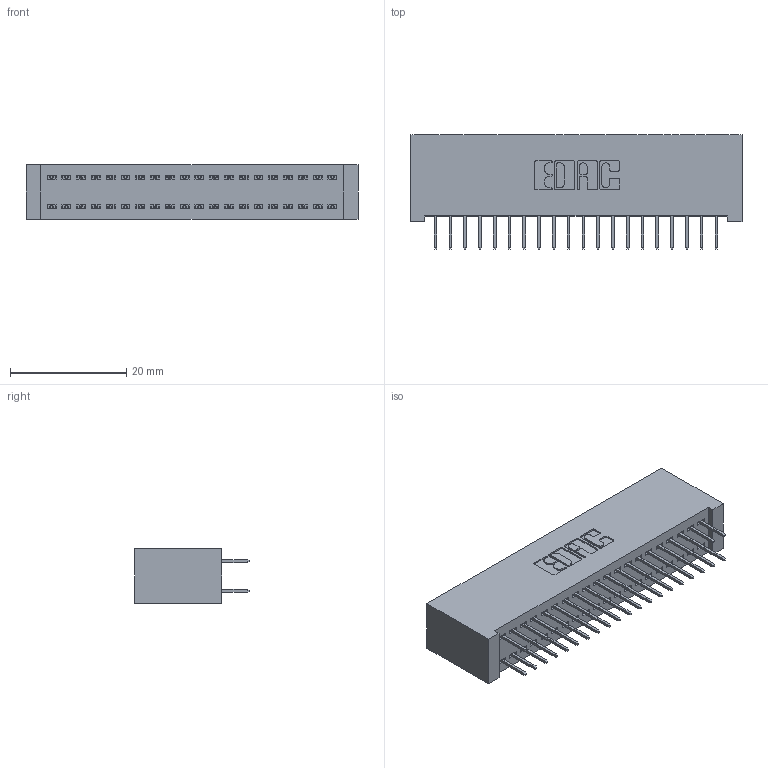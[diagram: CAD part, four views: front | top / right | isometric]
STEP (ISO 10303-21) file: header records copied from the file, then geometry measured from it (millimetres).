
FILE_DESCRIPTION (( 'STEP AP203' ), '1' );
FILE_NAME ('342-040-524-201.STEP', '2018-08-12T00:16:53', ( '' ), ( '' ), 'SwSTEP 2.0', 'SolidWorks 2016', '' );
FILE_SCHEMA (( 'CONFIG_CONTROL_DESIGN' ));
Length unit declared in the file: inch
Products named in the file (3): 345-292-001_345-293-124; 342-040-524-201; 342 Part_Lugless
Assembly tree (41 placements, depth 2):
  342-040-524-201
    342 Part_Lugless
    345-292-001_345-293-124  x40
Bounding box: 57.05 x 19.69 x 9.4 mm (x, y, z)
Volume: 5400.6 mm3; surface area: 8537.6 mm2
Topology: 41 solids, 41 shells, 2342 faces, 6635 edges, 4262 vertices
Faces by surface type: plane 1742, cylinder 600
Entity records: 15377 total; most frequent: CARTESIAN_POINT 2570, ORIENTED_EDGE 2506, DIRECTION 2229, EDGE_CURVE 1253, LINE 1137, VECTOR 1137, VERTEX_POINT 830, AXIS2_PLACEMENT_3D 546
